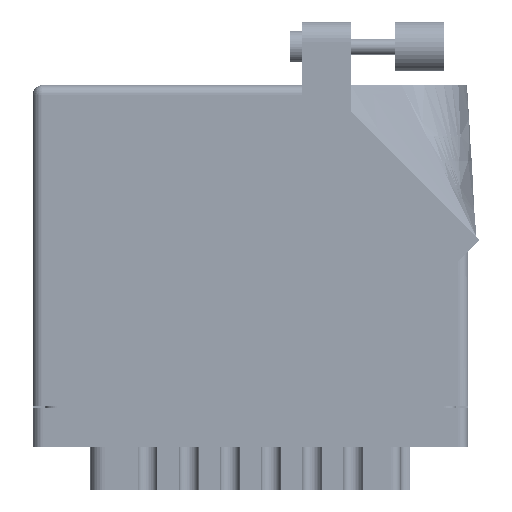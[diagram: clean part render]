
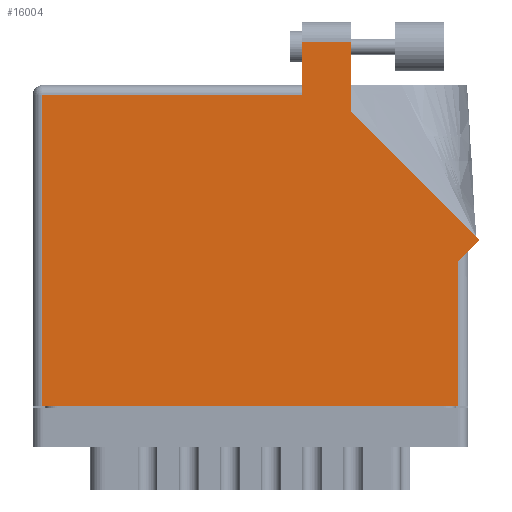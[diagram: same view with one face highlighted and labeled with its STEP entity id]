
A CAD part, front view. The second image highlights one B-rep face of the part: STEP entity #16004.
In plain terms, the highlighted face is planar.
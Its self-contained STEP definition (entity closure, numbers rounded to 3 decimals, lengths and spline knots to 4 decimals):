
#1365 = EDGE_CURVE ( 'NONE', #74328, #46928, #28747, .T. ) ;
#4650 = LINE ( 'NONE', #59441, #7019 ) ;
#7019 = VECTOR ( 'NONE', #14773, 39.3701 ) ;
#7465 = CARTESIAN_POINT ( 'NONE',  ( 0.062, 1.968, 0. ) ) ;
#10399 = ORIENTED_EDGE ( 'NONE', *, *, #92718, .T. ) ;
#10771 = VECTOR ( 'NONE', #83242, 39.3701 ) ;
#11094 = DIRECTION ( 'NONE',  ( -1., 0., 0. ) ) ;
#12539 = DIRECTION ( 'NONE',  ( -0.707, 0.707, 0. ) ) ;
#14773 = DIRECTION ( 'NONE',  ( 1., 0., 0. ) ) ;
#15479 = VERTEX_POINT ( 'NONE', #90804 ) ;
#16004 = ADVANCED_FACE ( 'NONE', ( #17653 ), #20495, .F. ) ;
#17302 = LINE ( 'NONE', #57849, #54710 ) ;
#17653 = FACE_OUTER_BOUND ( 'NONE', #78503, .T. ) ;
#17704 = LINE ( 'NONE', #68889, #10771 ) ;
#19480 = LINE ( 'NONE', #71686, #27727 ) ;
#19822 = DIRECTION ( 'NONE',  ( -1., 0., 0. ) ) ;
#19952 = LINE ( 'NONE', #93970, #41081 ) ;
#20020 = CARTESIAN_POINT ( 'NONE',  ( 2.693, 0.918, 0. ) ) ;
#20123 = VERTEX_POINT ( 'NONE', #52115 ) ;
#20495 = PLANE ( 'NONE',  #81690 ) ;
#20798 = DIRECTION ( 'NONE',  ( 0., 0., -1. ) ) ;
#24323 = EDGE_CURVE ( 'NONE', #46928, #20123, #17302, .T. ) ;
#25797 = DIRECTION ( 'NONE',  ( 0., 1., 0. ) ) ;
#25948 = VECTOR ( 'NONE', #94185, 39.3701 ) ;
#27727 = VECTOR ( 'NONE', #19822, 39.3701 ) ;
#28747 = LINE ( 'NONE', #89391, #46199 ) ;
#28798 = ORIENTED_EDGE ( 'NONE', *, *, #24323, .T. ) ;
#28986 = VERTEX_POINT ( 'NONE', #32241 ) ;
#29980 = VERTEX_POINT ( 'NONE', #51990 ) ;
#31011 = LINE ( 'NONE', #31396, #46156 ) ;
#31396 = CARTESIAN_POINT ( 'NONE',  ( 1.705, 2.03, 0. ) ) ;
#32241 = CARTESIAN_POINT ( 'NONE',  ( 1.705, 2.305, 0. ) ) ;
#35255 = ORIENTED_EDGE ( 'NONE', *, *, #65888, .T. ) ;
#40764 = CARTESIAN_POINT ( 'NONE',  ( 0., 2.03, 0. ) ) ;
#41081 = VECTOR ( 'NONE', #57788, 39.3701 ) ;
#41122 = CARTESIAN_POINT ( 'NONE',  ( 2.693, 0.98, 0. ) ) ;
#43671 = CARTESIAN_POINT ( 'NONE',  ( 2.693, 0., 0. ) ) ;
#45061 = VECTOR ( 'NONE', #25797, 39.3701 ) ;
#46156 = VECTOR ( 'NONE', #54843, 39.3701 ) ;
#46199 = VECTOR ( 'NONE', #59699, 39.3701 ) ;
#46928 = VERTEX_POINT ( 'NONE', #73371 ) ;
#48067 = ORIENTED_EDGE ( 'NONE', *, *, #58058, .T. ) ;
#51313 = EDGE_CURVE ( 'NONE', #29980, #86868, #4650, .T. ) ;
#51990 = CARTESIAN_POINT ( 'NONE',  ( 0.062, 0., 0. ) ) ;
#52115 = CARTESIAN_POINT ( 'NONE',  ( 2.012, 1.8644, 0. ) ) ;
#54101 = ORIENTED_EDGE ( 'NONE', *, *, #63690, .T. ) ;
#54710 = VECTOR ( 'NONE', #12539, 39.3701 ) ;
#54843 = DIRECTION ( 'NONE',  ( 0., -1., 0. ) ) ;
#57788 = DIRECTION ( 'NONE',  ( 0., -1., 0. ) ) ;
#57842 = EDGE_CURVE ( 'NONE', #20123, #96338, #17704, .T. ) ;
#57849 = CARTESIAN_POINT ( 'NONE',  ( 2.8257, 1.0507, 0. ) ) ;
#58058 = EDGE_CURVE ( 'NONE', #92649, #29980, #19952, .T. ) ;
#59441 = CARTESIAN_POINT ( 'NONE',  ( 0., 0., 0. ) ) ;
#59699 = DIRECTION ( 'NONE',  ( 0.707, 0.707, 0. ) ) ;
#62191 = EDGE_CURVE ( 'NONE', #15479, #92649, #19480, .T. ) ;
#63690 = EDGE_CURVE ( 'NONE', #86868, #74328, #85768, .T. ) ;
#65623 = ORIENTED_EDGE ( 'NONE', *, *, #62191, .T. ) ;
#65888 = EDGE_CURVE ( 'NONE', #96338, #28986, #78369, .T. ) ;
#68889 = CARTESIAN_POINT ( 'NONE',  ( 2.012, 1.8644, 0. ) ) ;
#71686 = CARTESIAN_POINT ( 'NONE',  ( 0., 1.968, 0. ) ) ;
#72961 = ORIENTED_EDGE ( 'NONE', *, *, #57842, .T. ) ;
#73371 = CARTESIAN_POINT ( 'NONE',  ( 2.8257, 1.0507, 0. ) ) ;
#74328 = VERTEX_POINT ( 'NONE', #20020 ) ;
#78369 = LINE ( 'NONE', #94824, #25948 ) ;
#78503 = EDGE_LOOP ( 'NONE', ( #72961, #35255, #10399, #65623, #48067, #92766, #54101, #87264, #28798 ) ) ;
#80878 = CARTESIAN_POINT ( 'NONE',  ( 2.012, 2.305, 0. ) ) ;
#81690 = AXIS2_PLACEMENT_3D ( 'NONE', #40764, #20798, #11094 ) ;
#83242 = DIRECTION ( 'NONE',  ( 0., 1., 0. ) ) ;
#85768 = LINE ( 'NONE', #41122, #45061 ) ;
#86868 = VERTEX_POINT ( 'NONE', #43671 ) ;
#87264 = ORIENTED_EDGE ( 'NONE', *, *, #1365, .T. ) ;
#89391 = CARTESIAN_POINT ( 'NONE',  ( 2.755, 0.98, 0. ) ) ;
#90804 = CARTESIAN_POINT ( 'NONE',  ( 1.705, 1.968, 0. ) ) ;
#92649 = VERTEX_POINT ( 'NONE', #7465 ) ;
#92718 = EDGE_CURVE ( 'NONE', #28986, #15479, #31011, .T. ) ;
#92766 = ORIENTED_EDGE ( 'NONE', *, *, #51313, .T. ) ;
#93970 = CARTESIAN_POINT ( 'NONE',  ( 0.062, 0., 0. ) ) ;
#94185 = DIRECTION ( 'NONE',  ( -1., 0., 0. ) ) ;
#94824 = CARTESIAN_POINT ( 'NONE',  ( 1.705, 2.305, 0. ) ) ;
#96338 = VERTEX_POINT ( 'NONE', #80878 ) ;
